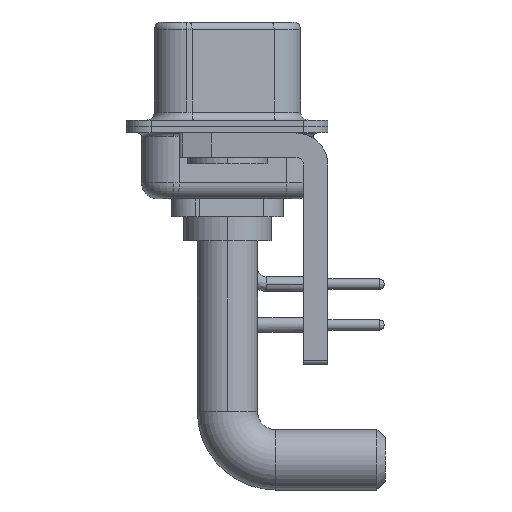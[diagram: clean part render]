
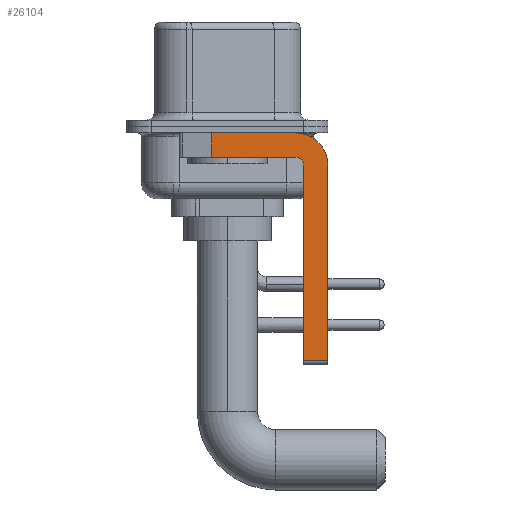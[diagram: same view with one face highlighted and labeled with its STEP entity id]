
A CAD part, left-side view. The second image highlights one B-rep face of the part: STEP entity #26104.
In plain terms, the highlighted planar face has unit normal (-1, 0, 0).
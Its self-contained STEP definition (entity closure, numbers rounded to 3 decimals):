
#314 = ORIENTED_EDGE ( 'NONE', *, *, #7556, .F. ) ;
#470 = CARTESIAN_POINT ( 'NONE',  ( -2.9, -4.25, -1.9 ) ) ;
#512 = VERTEX_POINT ( 'NONE', #7051 ) ;
#883 = EDGE_CURVE ( 'NONE', #13298, #925, #10884, .T. ) ;
#925 = VERTEX_POINT ( 'NONE', #16202 ) ;
#990 = CARTESIAN_POINT ( 'NONE',  ( -2.9, -4.25, -1.9 ) ) ;
#1198 = DIRECTION ( 'NONE',  ( 0., -1., 0. ) ) ;
#2238 = CARTESIAN_POINT ( 'NONE',  ( -2.9, -4.75, -14.8 ) ) ;
#2274 = CIRCLE ( 'NONE', #23143, 2. ) ;
#2336 = DIRECTION ( 'NONE',  ( 0., 0., -1. ) ) ;
#2354 = EDGE_CURVE ( 'NONE', #10824, #20927, #17156, .T. ) ;
#2991 = EDGE_CURVE ( 'NONE', #20927, #15998, #14777, .T. ) ;
#3186 = ORIENTED_EDGE ( 'NONE', *, *, #25963, .T. ) ;
#3413 = CARTESIAN_POINT ( 'NONE',  ( -2.9, -4.75, -14.55 ) ) ;
#3554 = EDGE_CURVE ( 'NONE', #23156, #10824, #29206, .T. ) ;
#3947 = VECTOR ( 'NONE', #4078, 1000. ) ;
#3994 = ORIENTED_EDGE ( 'NONE', *, *, #26676, .F. ) ;
#4078 = DIRECTION ( 'NONE',  ( 0., -1., 0. ) ) ;
#4590 = CARTESIAN_POINT ( 'NONE',  ( -2.9, -4.25, -2.4 ) ) ;
#5320 = AXIS2_PLACEMENT_3D ( 'NONE', #4590, #22807, #6513 ) ;
#5889 = CARTESIAN_POINT ( 'NONE',  ( -2.9, -4.25, -2.4 ) ) ;
#6317 = ORIENTED_EDGE ( 'NONE', *, *, #2354, .F. ) ;
#6513 = DIRECTION ( 'NONE',  ( 0., 0., 1. ) ) ;
#6786 = CARTESIAN_POINT ( 'NONE',  ( -2.9, 0.978, -1.9 ) ) ;
#7051 = CARTESIAN_POINT ( 'NONE',  ( -2.9, -4.25, -0.4 ) ) ;
#7556 = EDGE_CURVE ( 'NONE', #512, #13298, #2274, .T. ) ;
#8203 = VECTOR ( 'NONE', #8908, 1000. ) ;
#8908 = DIRECTION ( 'NONE',  ( 0., 0., 1. ) ) ;
#9870 = VERTEX_POINT ( 'NONE', #16156 ) ;
#10824 = VERTEX_POINT ( 'NONE', #18999 ) ;
#10884 = LINE ( 'NONE', #24205, #10942 ) ;
#10942 = VECTOR ( 'NONE', #19900, 1000. ) ;
#11069 = CARTESIAN_POINT ( 'NONE',  ( -2.9, 0.978, -1.9 ) ) ;
#11192 = ORIENTED_EDGE ( 'NONE', *, *, #883, .F. ) ;
#11207 = LINE ( 'NONE', #16087, #3947 ) ;
#11272 = ORIENTED_EDGE ( 'NONE', *, *, #2991, .F. ) ;
#11675 = FACE_OUTER_BOUND ( 'NONE', #13111, .T. ) ;
#12032 = EDGE_CURVE ( 'NONE', #9870, #15998, #14259, .T. ) ;
#12709 = DIRECTION ( 'NONE',  ( 1., 0., 0. ) ) ;
#13111 = EDGE_LOOP ( 'NONE', ( #3994, #21128, #11272, #6317, #19165, #3186, #11192, #314 ) ) ;
#13298 = VERTEX_POINT ( 'NONE', #15077 ) ;
#13756 = CARTESIAN_POINT ( 'NONE',  ( -2.9, -4.25, -2.4 ) ) ;
#14259 = LINE ( 'NONE', #11069, #19276 ) ;
#14777 = LINE ( 'NONE', #990, #28530 ) ;
#15077 = CARTESIAN_POINT ( 'NONE',  ( -2.9, -6.25, -2.4 ) ) ;
#15836 = VECTOR ( 'NONE', #1198, 1000. ) ;
#15998 = VERTEX_POINT ( 'NONE', #6786 ) ;
#16087 = CARTESIAN_POINT ( 'NONE',  ( -2.9, 3., -0.4 ) ) ;
#16156 = CARTESIAN_POINT ( 'NONE',  ( -2.9, 0.978, -0.4 ) ) ;
#16202 = CARTESIAN_POINT ( 'NONE',  ( -2.9, -6.25, -14.55 ) ) ;
#16483 = DIRECTION ( 'NONE',  ( 0., 0., -1. ) ) ;
#16911 = CARTESIAN_POINT ( 'NONE',  ( -2.9, -4.25, -14.55 ) ) ;
#17156 = CIRCLE ( 'NONE', #5320, 0.5 ) ;
#18999 = CARTESIAN_POINT ( 'NONE',  ( -2.9, -4.75, -2.4 ) ) ;
#19165 = ORIENTED_EDGE ( 'NONE', *, *, #3554, .F. ) ;
#19276 = VECTOR ( 'NONE', #16483, 1000. ) ;
#19900 = DIRECTION ( 'NONE',  ( 0., 0., -1. ) ) ;
#20066 = AXIS2_PLACEMENT_3D ( 'NONE', #13756, #27224, #2336 ) ;
#20927 = VERTEX_POINT ( 'NONE', #470 ) ;
#21128 = ORIENTED_EDGE ( 'NONE', *, *, #12032, .T. ) ;
#22807 = DIRECTION ( 'NONE',  ( -1., 0., 0. ) ) ;
#23143 = AXIS2_PLACEMENT_3D ( 'NONE', #5889, #12709, #24533 ) ;
#23156 = VERTEX_POINT ( 'NONE', #3413 ) ;
#23572 = LINE ( 'NONE', #16911, #15836 ) ;
#24205 = CARTESIAN_POINT ( 'NONE',  ( -2.9, -6.25, -2.4 ) ) ;
#24533 = DIRECTION ( 'NONE',  ( 0., 0., -1. ) ) ;
#24868 = PLANE ( 'NONE',  #20066 ) ;
#25963 = EDGE_CURVE ( 'NONE', #23156, #925, #23572, .T. ) ;
#26104 = ADVANCED_FACE ( 'NONE', ( #11675 ), #24868, .F. ) ;
#26676 = EDGE_CURVE ( 'NONE', #9870, #512, #11207, .T. ) ;
#27224 = DIRECTION ( 'NONE',  ( 1., 0., 0. ) ) ;
#28530 = VECTOR ( 'NONE', #28681, 1000. ) ;
#28681 = DIRECTION ( 'NONE',  ( 0., 1., 0. ) ) ;
#29206 = LINE ( 'NONE', #2238, #8203 ) ;
